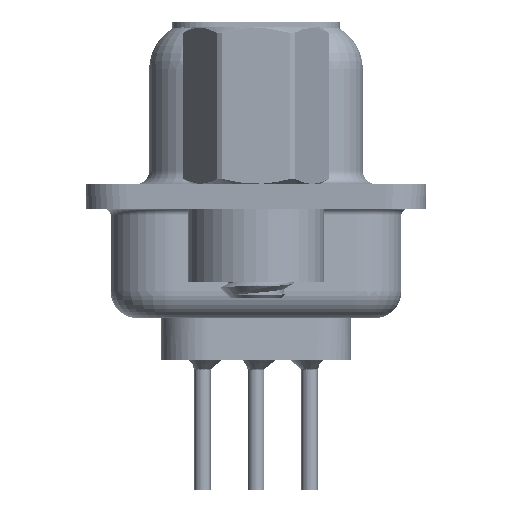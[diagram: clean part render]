
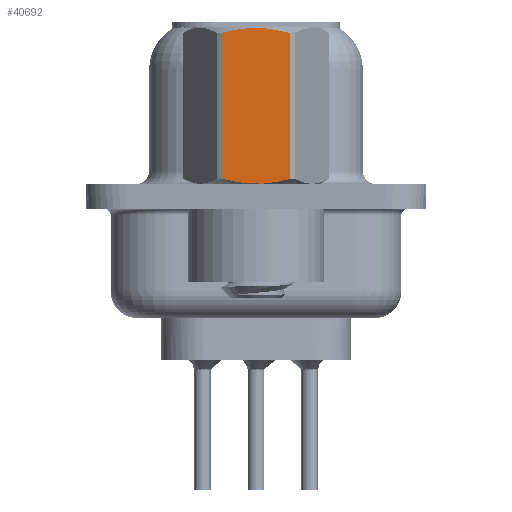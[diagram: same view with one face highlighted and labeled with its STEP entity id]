
A CAD part, left-side view. The second image highlights one B-rep face of the part: STEP entity #40692.
In plain terms, the highlighted planar face has unit normal (-1, 0, 0).
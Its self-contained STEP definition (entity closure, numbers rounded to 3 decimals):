
#2714 = B_SPLINE_CURVE_WITH_KNOTS ( 'NONE', 3,
 ( #38072, #18371, #42788, #22054, #34406, #38337, #29944, #26271, #9956, #38592 ),
 .UNSPECIFIED., .F., .F.,
 ( 4, 2, 2, 2, 4 ),
 ( 0.001, 0.002, 0.002, 0.003, 0.004 ),
 .UNSPECIFIED. ) ;
#3985 = DIRECTION ( 'NONE',  ( -1., 0., 0. ) ) ;
#5669 = CARTESIAN_POINT ( 'NONE',  ( -2.381, 0.428, 0.485 ) ) ;
#6494 = EDGE_CURVE ( 'NONE', #35308, #14388, #2714, .T. ) ;
#7241 = LINE ( 'NONE', #11484, #31362 ) ;
#7523 = ORIENTED_EDGE ( 'NONE', *, *, #41879, .T. ) ;
#7908 = FACE_OUTER_BOUND ( 'NONE', #27380, .T. ) ;
#9908 = CARTESIAN_POINT ( 'NONE',  ( -2.381, -1.066, 0.596 ) ) ;
#9956 = CARTESIAN_POINT ( 'NONE',  ( -2.381, 1.065, 6.104 ) ) ;
#10164 = CARTESIAN_POINT ( 'NONE',  ( -2.381, -1.273, 0.652 ) ) ;
#10430 = CARTESIAN_POINT ( 'NONE',  ( -2.381, -0.215, 0.468 ) ) ;
#11484 = CARTESIAN_POINT ( 'NONE',  ( -2.381, 1.273, 3.792 ) ) ;
#13851 = CARTESIAN_POINT ( 'NONE',  ( -2.381, -0.432, 0.485 ) ) ;
#14388 = VERTEX_POINT ( 'NONE', #21826 ) ;
#15137 = DIRECTION ( 'NONE',  ( 0., 0., -1. ) ) ;
#17807 = CARTESIAN_POINT ( 'NONE',  ( -2.381, 0.215, 0.468 ) ) ;
#17828 = B_SPLINE_CURVE_WITH_KNOTS ( 'NONE', 3,
 ( #26741, #46182, #33573, #5669, #17807, #10430, #13851, #45928, #9908, #10164 ),
 .UNSPECIFIED., .F., .F.,
 ( 4, 2, 2, 2, 4 ),
 ( 0.003, 0.003, 0.004, 0.004, 0.005 ),
 .UNSPECIFIED. ) ;
#18371 = CARTESIAN_POINT ( 'NONE',  ( -2.381, -1.066, 6.104 ) ) ;
#19774 = CARTESIAN_POINT ( 'NONE',  ( -2.381, 1.273, 0.652 ) ) ;
#21756 = VERTEX_POINT ( 'NONE', #27546 ) ;
#21826 = CARTESIAN_POINT ( 'NONE',  ( -2.381, 1.273, 6.048 ) ) ;
#22054 = CARTESIAN_POINT ( 'NONE',  ( -2.381, -0.432, 6.215 ) ) ;
#23989 = ORIENTED_EDGE ( 'NONE', *, *, #45015, .T. ) ;
#24998 = EDGE_CURVE ( 'NONE', #45339, #21756, #17828, .T. ) ;
#26271 = CARTESIAN_POINT ( 'NONE',  ( -2.381, 0.853, 6.151 ) ) ;
#26741 = CARTESIAN_POINT ( 'NONE',  ( -2.381, 1.273, 0.652 ) ) ;
#26765 = LINE ( 'NONE', #42767, #49120 ) ;
#27380 = EDGE_LOOP ( 'NONE', ( #39096, #23989, #45815, #7523 ) ) ;
#27546 = CARTESIAN_POINT ( 'NONE',  ( -2.381, -1.273, 0.652 ) ) ;
#27950 = CARTESIAN_POINT ( 'NONE',  ( -2.381, 1.375, -3.75 ) ) ;
#29944 = CARTESIAN_POINT ( 'NONE',  ( -2.381, 0.428, 6.215 ) ) ;
#31255 = AXIS2_PLACEMENT_3D ( 'NONE', #27950, #3985, #48399 ) ;
#31362 = VECTOR ( 'NONE', #15137, 1000. ) ;
#32387 = PLANE ( 'NONE',  #31255 ) ;
#33573 = CARTESIAN_POINT ( 'NONE',  ( -2.381, 0.853, 0.549 ) ) ;
#34406 = CARTESIAN_POINT ( 'NONE',  ( -2.381, -0.215, 6.232 ) ) ;
#35308 = VERTEX_POINT ( 'NONE', #46617 ) ;
#38072 = CARTESIAN_POINT ( 'NONE',  ( -2.381, -1.273, 6.048 ) ) ;
#38337 = CARTESIAN_POINT ( 'NONE',  ( -2.381, 0.215, 6.232 ) ) ;
#38592 = CARTESIAN_POINT ( 'NONE',  ( -2.381, 1.273, 6.048 ) ) ;
#39096 = ORIENTED_EDGE ( 'NONE', *, *, #24998, .T. ) ;
#40064 = DIRECTION ( 'NONE',  ( 0., 0., 1. ) ) ;
#40692 = ADVANCED_FACE ( 'NONE', ( #7908 ), #32387, .T. ) ;
#41879 = EDGE_CURVE ( 'NONE', #14388, #45339, #7241, .T. ) ;
#42767 = CARTESIAN_POINT ( 'NONE',  ( -2.381, -1.273, 3.792 ) ) ;
#42788 = CARTESIAN_POINT ( 'NONE',  ( -2.381, -0.858, 6.15 ) ) ;
#45015 = EDGE_CURVE ( 'NONE', #21756, #35308, #26765, .T. ) ;
#45339 = VERTEX_POINT ( 'NONE', #19774 ) ;
#45815 = ORIENTED_EDGE ( 'NONE', *, *, #6494, .T. ) ;
#45928 = CARTESIAN_POINT ( 'NONE',  ( -2.381, -0.858, 0.55 ) ) ;
#46182 = CARTESIAN_POINT ( 'NONE',  ( -2.381, 1.065, 0.596 ) ) ;
#46617 = CARTESIAN_POINT ( 'NONE',  ( -2.381, -1.273, 6.048 ) ) ;
#48399 = DIRECTION ( 'NONE',  ( 0., -1., 0. ) ) ;
#49120 = VECTOR ( 'NONE', #40064, 1000. ) ;
